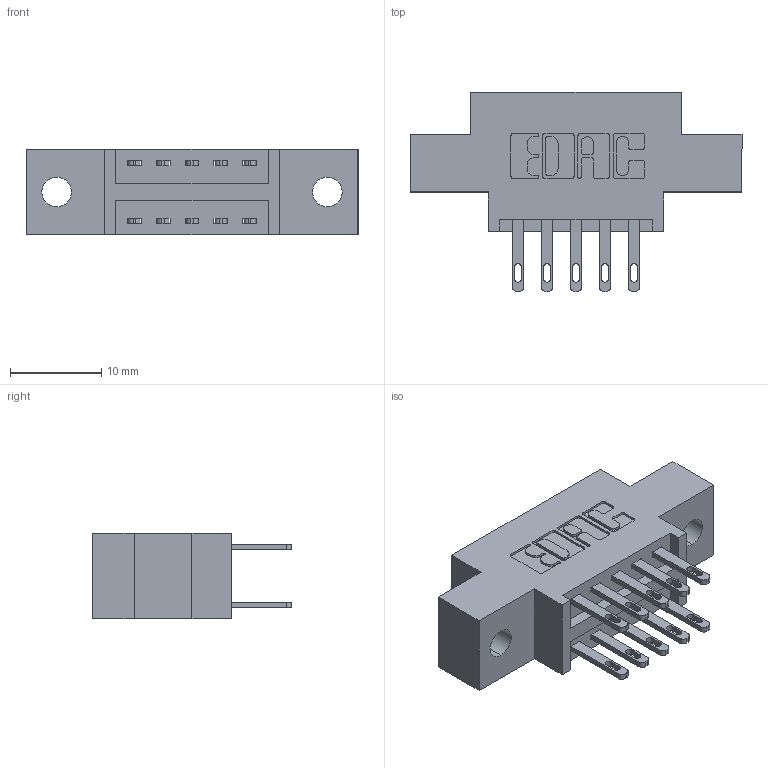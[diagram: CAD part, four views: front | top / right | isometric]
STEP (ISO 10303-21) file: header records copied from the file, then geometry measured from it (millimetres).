
FILE_DESCRIPTION (( 'STEP AP203' ), '1' );
FILE_NAME ('896-010-500-802.STEP', '2021-07-27T14:27:10', ( '' ), ( '' ), 'SwSTEP 2.0', 'SolidWorks 2020', '' );
FILE_SCHEMA (( 'CONFIG_CONTROL_DESIGN' ));
Length unit declared in the file: inch
Products named in the file (3): 345-292-001_345-293-100; 896-010-500-802; 846 Part_0.170 Offset - 0.128 Dia
Assembly tree (11 placements, depth 2):
  896-010-500-802
    846 Part_0.170 Offset - 0.128 Dia
    345-292-001_345-293-100  x10
Bounding box: 36.45 x 21.84 x 9.4 mm (x, y, z)
Volume: 3106.1 mm3; surface area: 3703.1 mm2
Topology: 11 solids, 11 shells, 606 faces, 1811 edges, 1206 vertices
Faces by surface type: plane 370, cylinder 236
Entity records: 8309 total; most frequent: CARTESIAN_POINT 1420, ORIENTED_EDGE 1354, DIRECTION 1305, EDGE_CURVE 677, LINE 521, VECTOR 521, VERTEX_POINT 450, AXIS2_PLACEMENT_3D 392
